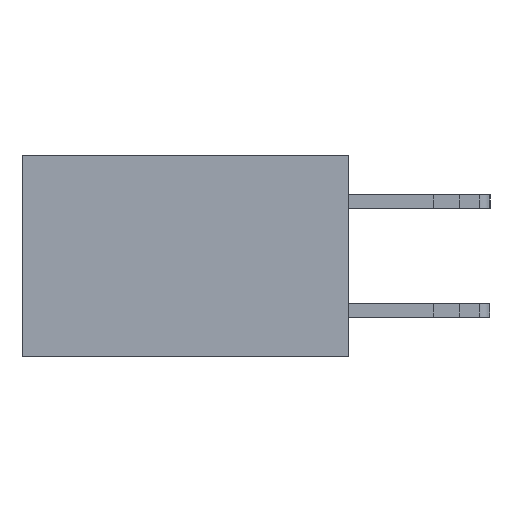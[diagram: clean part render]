
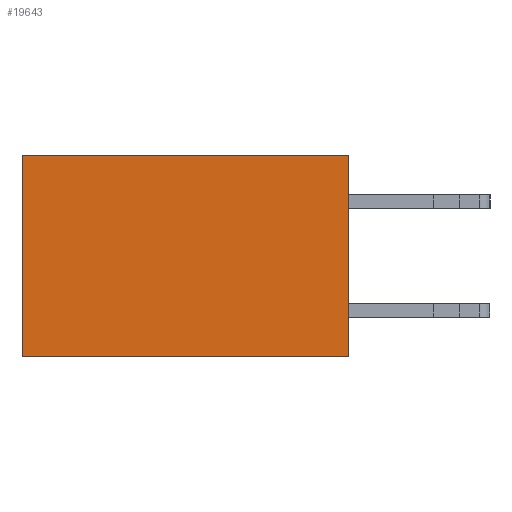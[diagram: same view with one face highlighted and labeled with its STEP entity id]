
A CAD part, left-side view. The second image highlights one B-rep face of the part: STEP entity #19643.
In plain terms, the highlighted planar face has unit normal (-1, 0, 0).
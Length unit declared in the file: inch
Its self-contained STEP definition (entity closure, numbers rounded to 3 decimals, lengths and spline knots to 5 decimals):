
#207 = FACE_OUTER_BOUND ( 'NONE', #19649, .T. ) ;
#243 = CARTESIAN_POINT ( 'NONE',  ( 0.298, 0., 0. ) ) ;
#1002 = CARTESIAN_POINT ( 'NONE',  ( 0.298, 0., -0.37 ) ) ;
#1538 = LINE ( 'NONE', #3617, #23430 ) ;
#2143 = CARTESIAN_POINT ( 'NONE',  ( 0.298, 0.6, 0. ) ) ;
#2966 = VECTOR ( 'NONE', #17245, 39.37008 ) ;
#3076 = VERTEX_POINT ( 'NONE', #2143 ) ;
#3617 = CARTESIAN_POINT ( 'NONE',  ( 0.298, 0.6, 0. ) ) ;
#3823 = LINE ( 'NONE', #243, #8436 ) ;
#6128 = DIRECTION ( 'NONE',  ( 0., 1., 0. ) ) ;
#6487 = VERTEX_POINT ( 'NONE', #9666 ) ;
#6985 = ORIENTED_EDGE ( 'NONE', *, *, #10902, .T. ) ;
#7007 = CARTESIAN_POINT ( 'NONE',  ( 0.298, 0., 0. ) ) ;
#8436 = VECTOR ( 'NONE', #6128, 39.37008 ) ;
#9301 = VECTOR ( 'NONE', #14711, 39.37008 ) ;
#9666 = CARTESIAN_POINT ( 'NONE',  ( 0.298, 0., -0.37 ) ) ;
#9791 = AXIS2_PLACEMENT_3D ( 'NONE', #11258, #24717, #13233 ) ;
#9859 = VERTEX_POINT ( 'NONE', #10930 ) ;
#10902 = EDGE_CURVE ( 'NONE', #3076, #9859, #1538, .T. ) ;
#10930 = CARTESIAN_POINT ( 'NONE',  ( 0.298, 0.6, -0.37 ) ) ;
#11258 = CARTESIAN_POINT ( 'NONE',  ( 0.298, 0., 0. ) ) ;
#13233 = DIRECTION ( 'NONE',  ( 0., 0., -1. ) ) ;
#13528 = EDGE_CURVE ( 'NONE', #16129, #6487, #18603, .T. ) ;
#14644 = EDGE_CURVE ( 'NONE', #16129, #3076, #3823, .T. ) ;
#14711 = DIRECTION ( 'NONE',  ( 0., 1., 0. ) ) ;
#15140 = LINE ( 'NONE', #1002, #9301 ) ;
#15434 = EDGE_CURVE ( 'NONE', #6487, #9859, #15140, .T. ) ;
#16129 = VERTEX_POINT ( 'NONE', #7007 ) ;
#17245 = DIRECTION ( 'NONE',  ( 0., 0., -1. ) ) ;
#17269 = DIRECTION ( 'NONE',  ( 0., 0., -1. ) ) ;
#18508 = ORIENTED_EDGE ( 'NONE', *, *, #15434, .F. ) ;
#18603 = LINE ( 'NONE', #22902, #2966 ) ;
#18789 = ORIENTED_EDGE ( 'NONE', *, *, #14644, .T. ) ;
#19490 = ORIENTED_EDGE ( 'NONE', *, *, #13528, .F. ) ;
#19643 = ADVANCED_FACE ( 'NONE', ( #207 ), #20968, .F. ) ;
#19649 = EDGE_LOOP ( 'NONE', ( #6985, #18508, #19490, #18789 ) ) ;
#20968 = PLANE ( 'NONE',  #9791 ) ;
#22902 = CARTESIAN_POINT ( 'NONE',  ( 0.298, 0., 0. ) ) ;
#23430 = VECTOR ( 'NONE', #17269, 39.37008 ) ;
#24717 = DIRECTION ( 'NONE',  ( 1., 0., 0. ) ) ;
